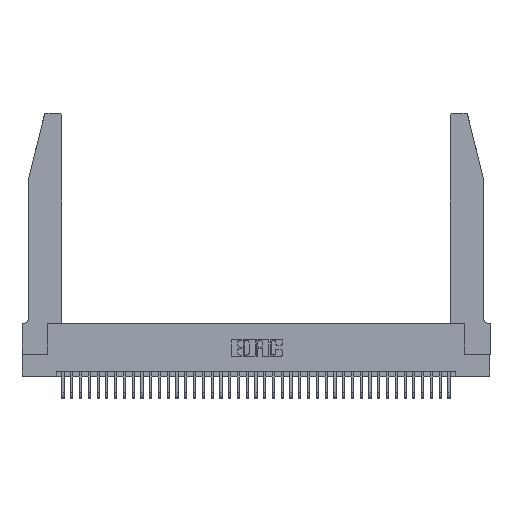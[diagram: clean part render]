
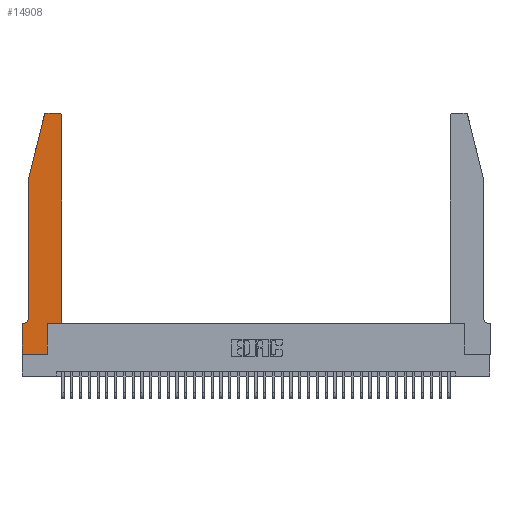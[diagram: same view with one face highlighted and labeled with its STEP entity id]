
A CAD part, top view. The second image highlights one B-rep face of the part: STEP entity #14908.
In plain terms, the highlighted planar face has unit normal (0, 0, 1).
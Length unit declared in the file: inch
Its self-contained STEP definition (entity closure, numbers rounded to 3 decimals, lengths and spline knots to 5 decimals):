
#93 = VERTEX_POINT ( 'NONE', #14723 ) ;
#640 = CARTESIAN_POINT ( 'NONE',  ( 0.2865, 0.35, 0.37 ) ) ;
#769 = VECTOR ( 'NONE', #21435, 39.37008 ) ;
#1041 = VECTOR ( 'NONE', #22377, 39.37008 ) ;
#1710 = LINE ( 'NONE', #6511, #8650 ) ;
#2315 = VERTEX_POINT ( 'NONE', #10938 ) ;
#2685 = CARTESIAN_POINT ( 'NONE',  ( 0.4205, 2.72, 0.37 ) ) ;
#3099 = EDGE_CURVE ( 'NONE', #93, #14316, #31805, .T. ) ;
#3242 = CARTESIAN_POINT ( 'NONE',  ( 0.4505, 0.35, 0.37 ) ) ;
#3294 = EDGE_CURVE ( 'NONE', #20033, #4221, #1710, .T. ) ;
#3338 = EDGE_CURVE ( 'NONE', #10034, #34268, #30430, .T. ) ;
#4221 = VERTEX_POINT ( 'NONE', #10942 ) ;
#4563 = CARTESIAN_POINT ( 'NONE',  ( 0.0755, 2., 0.37 ) ) ;
#5412 = CARTESIAN_POINT ( 'NONE',  ( 0.4505, 0.35, 0.37 ) ) ;
#5465 = CARTESIAN_POINT ( 'NONE',  ( 0.0755, 2., 0.37 ) ) ;
#5658 = DIRECTION ( 'NONE',  ( 1., 0., 0. ) ) ;
#5714 = ORIENTED_EDGE ( 'NONE', *, *, #20685, .T. ) ;
#6511 = CARTESIAN_POINT ( 'NONE',  ( 0., 0., 0.37 ) ) ;
#7282 = CARTESIAN_POINT ( 'NONE',  ( 0.2865, 0., 0.37 ) ) ;
#8650 = VECTOR ( 'NONE', #18350, 39.37008 ) ;
#8670 = VECTOR ( 'NONE', #12662, 39.37008 ) ;
#9255 = EDGE_LOOP ( 'NONE', ( #33147, #14776, #14343, #25601, #10169, #12806, #9628, #10866, #15793, #11770, #30747, #5714 ) ) ;
#9490 = CARTESIAN_POINT ( 'NONE',  ( 0.0755, 2., 0.37 ) ) ;
#9628 = ORIENTED_EDGE ( 'NONE', *, *, #3294, .T. ) ;
#9698 = CARTESIAN_POINT ( 'NONE',  ( 0.0055, 0.35, 0.37 ) ) ;
#9729 = CARTESIAN_POINT ( 'NONE',  ( 0.4505, 0.35, 0.37 ) ) ;
#10034 = VERTEX_POINT ( 'NONE', #7282 ) ;
#10169 = ORIENTED_EDGE ( 'NONE', *, *, #15523, .T. ) ;
#10866 = ORIENTED_EDGE ( 'NONE', *, *, #32431, .T. ) ;
#10938 = CARTESIAN_POINT ( 'NONE',  ( 0.4505, 2.72, 0.37 ) ) ;
#10942 = CARTESIAN_POINT ( 'NONE',  ( 0., 0., 0.37 ) ) ;
#11613 = VERTEX_POINT ( 'NONE', #36561 ) ;
#11770 = ORIENTED_EDGE ( 'NONE', *, *, #25435, .T. ) ;
#11982 = CARTESIAN_POINT ( 'NONE',  ( 0.2865, 0.35, 0.37 ) ) ;
#12395 = PLANE ( 'NONE',  #35599 ) ;
#12503 = CARTESIAN_POINT ( 'NONE',  ( 0., 0., 0.37 ) ) ;
#12662 = DIRECTION ( 'NONE',  ( 1., 0., 0. ) ) ;
#12776 = VECTOR ( 'NONE', #30507, 39.37008 ) ;
#12806 = ORIENTED_EDGE ( 'NONE', *, *, #23617, .T. ) ;
#13182 = AXIS2_PLACEMENT_3D ( 'NONE', #2685, #23457, #5658 ) ;
#13294 = DIRECTION ( 'NONE',  ( 0., 0., 1. ) ) ;
#13578 = VERTEX_POINT ( 'NONE', #26769 ) ;
#14316 = VERTEX_POINT ( 'NONE', #9490 ) ;
#14343 = ORIENTED_EDGE ( 'NONE', *, *, #3099, .T. ) ;
#14723 = CARTESIAN_POINT ( 'NONE',  ( 0.25487, 2.72718, 0.37 ) ) ;
#14776 = ORIENTED_EDGE ( 'NONE', *, *, #34005, .T. ) ;
#14908 = ADVANCED_FACE ( 'NONE', ( #32993 ), #12395, .T. ) ;
#14996 = DIRECTION ( 'NONE',  ( 0., 1., 0. ) ) ;
#15371 = DIRECTION ( 'NONE',  ( 0., 0., -1. ) ) ;
#15416 = DIRECTION ( 'NONE',  ( 1., 0., 0. ) ) ;
#15523 = EDGE_CURVE ( 'NONE', #38157, #17421, #20555, .T. ) ;
#15793 = ORIENTED_EDGE ( 'NONE', *, *, #3338, .T. ) ;
#16106 = VECTOR ( 'NONE', #37980, 39.37008 ) ;
#17421 = VERTEX_POINT ( 'NONE', #9698 ) ;
#18350 = DIRECTION ( 'NONE',  ( 0., -1., 0. ) ) ;
#19057 = EDGE_CURVE ( 'NONE', #13578, #11613, #28565, .T. ) ;
#19472 = CARTESIAN_POINT ( 'NONE',  ( 0.0755, 0.35, 0.37 ) ) ;
#20033 = VERTEX_POINT ( 'NONE', #20276 ) ;
#20276 = CARTESIAN_POINT ( 'NONE',  ( 0., 0.35, 0.37 ) ) ;
#20555 = CIRCLE ( 'NONE', #36121, 0.07 ) ;
#20685 = EDGE_CURVE ( 'NONE', #2315, #13578, #24812, .T. ) ;
#21435 = DIRECTION ( 'NONE',  ( 0., 1., 0. ) ) ;
#21528 = DIRECTION ( 'NONE',  ( 1., 0., 0. ) ) ;
#21540 = EDGE_CURVE ( 'NONE', #14316, #38157, #33441, .T. ) ;
#22242 = VECTOR ( 'NONE', #21528, 39.37008 ) ;
#22377 = DIRECTION ( 'NONE',  ( 0., -1., 0. ) ) ;
#23426 = AXIS2_PLACEMENT_3D ( 'NONE', #31058, #13294, #33992 ) ;
#23457 = DIRECTION ( 'NONE',  ( 0., 0., 1. ) ) ;
#23617 = EDGE_CURVE ( 'NONE', #17421, #20033, #32404, .T. ) ;
#23931 = VECTOR ( 'NONE', #14996, 39.37008 ) ;
#24647 = VECTOR ( 'NONE', #31161, 39.37008 ) ;
#24812 = CIRCLE ( 'NONE', #13182, 0.03 ) ;
#25435 = EDGE_CURVE ( 'NONE', #34268, #34220, #32264, .T. ) ;
#25601 = ORIENTED_EDGE ( 'NONE', *, *, #21540, .T. ) ;
#26769 = CARTESIAN_POINT ( 'NONE',  ( 0.4205, 2.75, 0.37 ) ) ;
#26975 = CARTESIAN_POINT ( 'NONE',  ( 0.0755, 0.42, 0.37 ) ) ;
#27560 = CARTESIAN_POINT ( 'NONE',  ( 0.2605, 2.75, 0.37 ) ) ;
#27970 = EDGE_CURVE ( 'NONE', #34220, #2315, #31707, .T. ) ;
#28565 = LINE ( 'NONE', #27560, #12776 ) ;
#30044 = LINE ( 'NONE', #12503, #22242 ) ;
#30173 = CARTESIAN_POINT ( 'NONE',  ( 0., 0.35, 0.37 ) ) ;
#30430 = LINE ( 'NONE', #640, #769 ) ;
#30507 = DIRECTION ( 'NONE',  ( -1., 0., 0. ) ) ;
#30747 = ORIENTED_EDGE ( 'NONE', *, *, #27970, .T. ) ;
#31058 = CARTESIAN_POINT ( 'NONE',  ( 0.284, 2.72, 0.37 ) ) ;
#31161 = DIRECTION ( 'NONE',  ( -1., 0., 0. ) ) ;
#31707 = LINE ( 'NONE', #3242, #23931 ) ;
#31805 = LINE ( 'NONE', #5465, #16106 ) ;
#32264 = LINE ( 'NONE', #9729, #8670 ) ;
#32404 = LINE ( 'NONE', #19472, #24647 ) ;
#32431 = EDGE_CURVE ( 'NONE', #4221, #10034, #30044, .T. ) ;
#32993 = FACE_OUTER_BOUND ( 'NONE', #9255, .T. ) ;
#33043 = CARTESIAN_POINT ( 'NONE',  ( 0.0055, 0.42, 0.37 ) ) ;
#33087 = DIRECTION ( 'NONE',  ( 0., 0., 1. ) ) ;
#33147 = ORIENTED_EDGE ( 'NONE', *, *, #19057, .T. ) ;
#33441 = LINE ( 'NONE', #4563, #1041 ) ;
#33992 = DIRECTION ( 'NONE',  ( 1., 0., 0. ) ) ;
#34005 = EDGE_CURVE ( 'NONE', #11613, #93, #38131, .T. ) ;
#34220 = VERTEX_POINT ( 'NONE', #5412 ) ;
#34268 = VERTEX_POINT ( 'NONE', #11982 ) ;
#35599 = AXIS2_PLACEMENT_3D ( 'NONE', #30173, #33087, #15416 ) ;
#35998 = DIRECTION ( 'NONE',  ( -1., 0., 0. ) ) ;
#36121 = AXIS2_PLACEMENT_3D ( 'NONE', #33043, #15371, #35998 ) ;
#36561 = CARTESIAN_POINT ( 'NONE',  ( 0.284, 2.75, 0.37 ) ) ;
#37980 = DIRECTION ( 'NONE',  ( -0.239, -0.971, 0. ) ) ;
#38131 = CIRCLE ( 'NONE', #23426, 0.03 ) ;
#38157 = VERTEX_POINT ( 'NONE', #26975 ) ;
